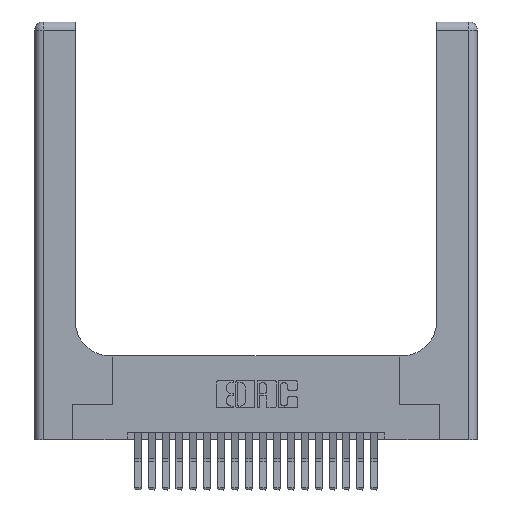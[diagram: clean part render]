
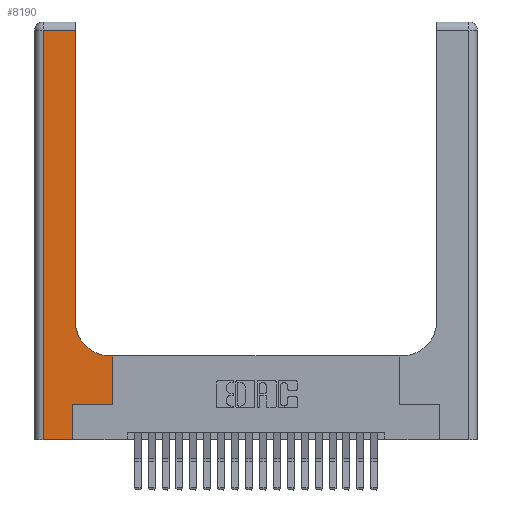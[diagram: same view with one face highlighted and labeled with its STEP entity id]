
A CAD part, top view. The second image highlights one B-rep face of the part: STEP entity #8190.
In plain terms, the highlighted planar face has unit normal (0, 0, 1).
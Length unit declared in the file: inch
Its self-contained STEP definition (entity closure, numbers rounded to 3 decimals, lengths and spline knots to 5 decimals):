
#28 = VECTOR ( 'NONE', #8898, 39.37008 ) ;
#237 = CIRCLE ( 'NONE', #8732, 0.25 ) ;
#964 = EDGE_CURVE ( 'NONE', #4676, #5911, #10465, .T. ) ;
#1864 = VECTOR ( 'NONE', #16106, 39.37008 ) ;
#2393 = LINE ( 'NONE', #17155, #2941 ) ;
#2486 = VECTOR ( 'NONE', #8800, 39.37008 ) ;
#2867 = VERTEX_POINT ( 'NONE', #16043 ) ;
#2897 = VERTEX_POINT ( 'NONE', #15106 ) ;
#2941 = VECTOR ( 'NONE', #17219, 39.37008 ) ;
#3186 = FACE_OUTER_BOUND ( 'NONE', #9408, .T. ) ;
#3322 = CARTESIAN_POINT ( 'NONE',  ( 0.5585, 0.25, 0.37 ) ) ;
#3635 = CARTESIAN_POINT ( 'NONE',  ( 0.5415, 0.85, 0.37 ) ) ;
#4676 = VERTEX_POINT ( 'NONE', #14933 ) ;
#5107 = LINE ( 'NONE', #22545, #7007 ) ;
#5228 = EDGE_CURVE ( 'NONE', #19319, #19640, #237, .T. ) ;
#5374 = DIRECTION ( 'NONE',  ( 0., 0., -1. ) ) ;
#5731 = PLANE ( 'NONE',  #17668 ) ;
#5911 = VERTEX_POINT ( 'NONE', #9704 ) ;
#6137 = CARTESIAN_POINT ( 'NONE',  ( 0., 2.94, 0.37 ) ) ;
#6470 = EDGE_CURVE ( 'NONE', #21774, #21038, #16015, .T. ) ;
#7007 = VECTOR ( 'NONE', #8354, 39.37008 ) ;
#7295 = EDGE_CURVE ( 'NONE', #19640, #21724, #18503, .T. ) ;
#7623 = LINE ( 'NONE', #8662, #18008 ) ;
#7758 = EDGE_CURVE ( 'NONE', #2897, #2867, #5107, .T. ) ;
#8190 = ADVANCED_FACE ( 'NONE', ( #3186 ), #5731, .F. ) ;
#8354 = DIRECTION ( 'NONE',  ( 0., 1., 0. ) ) ;
#8662 = CARTESIAN_POINT ( 'NONE',  ( 0.2915, 0.6, 0.37 ) ) ;
#8732 = AXIS2_PLACEMENT_3D ( 'NONE', #3635, #5374, #21186 ) ;
#8800 = DIRECTION ( 'NONE',  ( 1., 0., 0. ) ) ;
#8898 = DIRECTION ( 'NONE',  ( 0., -1., 0. ) ) ;
#9231 = VECTOR ( 'NONE', #15300, 39.37008 ) ;
#9408 = EDGE_LOOP ( 'NONE', ( #10890, #12553, #18138, #20111, #22542, #14720, #20760, #15002, #11375 ) ) ;
#9607 = CARTESIAN_POINT ( 'NONE',  ( 0.2915, 0.85, 0.37 ) ) ;
#9704 = CARTESIAN_POINT ( 'NONE',  ( 0.06, 0., 0.37 ) ) ;
#9753 = EDGE_CURVE ( 'NONE', #21724, #4676, #16732, .T. ) ;
#10058 = DIRECTION ( 'NONE',  ( -1., 0., 0. ) ) ;
#10465 = LINE ( 'NONE', #17574, #28 ) ;
#10718 = DIRECTION ( 'NONE',  ( 0., 0., -1. ) ) ;
#10742 = CARTESIAN_POINT ( 'NONE',  ( 0.5585, 0.25, 0.37 ) ) ;
#10890 = ORIENTED_EDGE ( 'NONE', *, *, #7295, .T. ) ;
#11375 = ORIENTED_EDGE ( 'NONE', *, *, #5228, .T. ) ;
#11546 = EDGE_CURVE ( 'NONE', #2867, #21774, #12069, .T. ) ;
#12069 = LINE ( 'NONE', #19245, #2486 ) ;
#12553 = ORIENTED_EDGE ( 'NONE', *, *, #9753, .T. ) ;
#14209 = DIRECTION ( 'NONE',  ( -1., 0., 0. ) ) ;
#14720 = ORIENTED_EDGE ( 'NONE', *, *, #11546, .T. ) ;
#14933 = CARTESIAN_POINT ( 'NONE',  ( 0.06, 2.94, 0.37 ) ) ;
#15002 = ORIENTED_EDGE ( 'NONE', *, *, #16485, .T. ) ;
#15106 = CARTESIAN_POINT ( 'NONE',  ( 0.269, 0., 0.37 ) ) ;
#15300 = DIRECTION ( 'NONE',  ( 0., 1., 0. ) ) ;
#16015 = LINE ( 'NONE', #10742, #1864 ) ;
#16043 = CARTESIAN_POINT ( 'NONE',  ( 0.269, 0.25, 0.37 ) ) ;
#16106 = DIRECTION ( 'NONE',  ( 0., 1., 0. ) ) ;
#16485 = EDGE_CURVE ( 'NONE', #21038, #19319, #7623, .T. ) ;
#16732 = LINE ( 'NONE', #6137, #20327 ) ;
#17155 = CARTESIAN_POINT ( 'NONE',  ( 0., 0., 0.37 ) ) ;
#17219 = DIRECTION ( 'NONE',  ( 1., 0., 0. ) ) ;
#17574 = CARTESIAN_POINT ( 'NONE',  ( 0.06, 3., 0.37 ) ) ;
#17627 = CARTESIAN_POINT ( 'NONE',  ( 0., 3., 0.37 ) ) ;
#17668 = AXIS2_PLACEMENT_3D ( 'NONE', #17627, #10718, #14209 ) ;
#18008 = VECTOR ( 'NONE', #21029, 39.37008 ) ;
#18138 = ORIENTED_EDGE ( 'NONE', *, *, #964, .T. ) ;
#18503 = LINE ( 'NONE', #18757, #9231 ) ;
#18757 = CARTESIAN_POINT ( 'NONE',  ( 0.2915, 3., 0.37 ) ) ;
#19158 = EDGE_CURVE ( 'NONE', #5911, #2897, #2393, .T. ) ;
#19245 = CARTESIAN_POINT ( 'NONE',  ( 0.269, 0.25, 0.37 ) ) ;
#19319 = VERTEX_POINT ( 'NONE', #19513 ) ;
#19513 = CARTESIAN_POINT ( 'NONE',  ( 0.5415, 0.6, 0.37 ) ) ;
#19640 = VERTEX_POINT ( 'NONE', #9607 ) ;
#20111 = ORIENTED_EDGE ( 'NONE', *, *, #19158, .T. ) ;
#20318 = CARTESIAN_POINT ( 'NONE',  ( 0.5585, 0.6, 0.37 ) ) ;
#20327 = VECTOR ( 'NONE', #10058, 39.37008 ) ;
#20760 = ORIENTED_EDGE ( 'NONE', *, *, #6470, .T. ) ;
#21029 = DIRECTION ( 'NONE',  ( -1., 0., 0. ) ) ;
#21038 = VERTEX_POINT ( 'NONE', #20318 ) ;
#21186 = DIRECTION ( 'NONE',  ( 1., 0., 0. ) ) ;
#21724 = VERTEX_POINT ( 'NONE', #22637 ) ;
#21774 = VERTEX_POINT ( 'NONE', #3322 ) ;
#22542 = ORIENTED_EDGE ( 'NONE', *, *, #7758, .T. ) ;
#22545 = CARTESIAN_POINT ( 'NONE',  ( 0.269, 0., 0.37 ) ) ;
#22637 = CARTESIAN_POINT ( 'NONE',  ( 0.2915, 2.94, 0.37 ) ) ;
